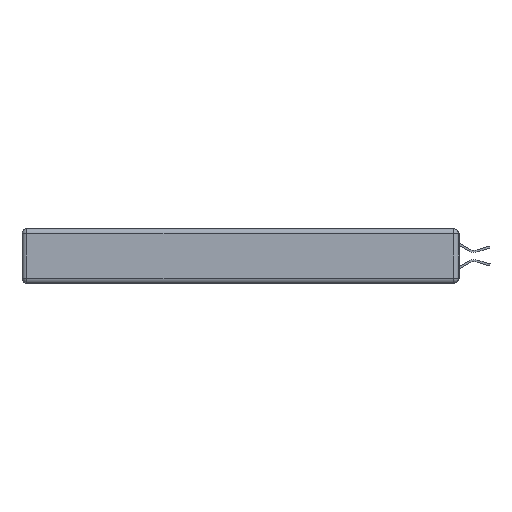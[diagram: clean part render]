
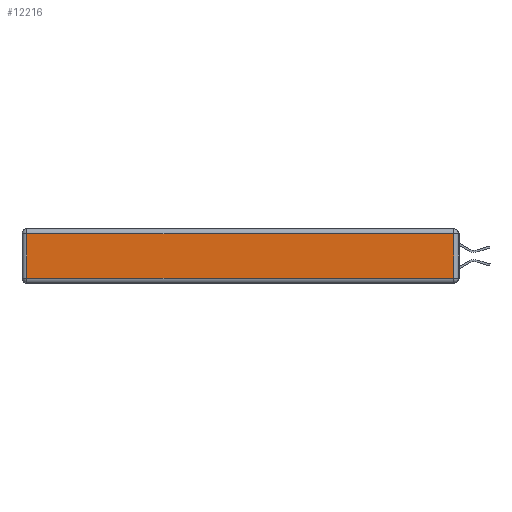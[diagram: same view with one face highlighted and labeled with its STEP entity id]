
A CAD part, left-side view. The second image highlights one B-rep face of the part: STEP entity #12216.
In plain terms, the highlighted planar face has unit normal (-1, 0, 0).
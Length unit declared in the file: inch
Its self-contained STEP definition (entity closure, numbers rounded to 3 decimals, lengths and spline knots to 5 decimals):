
#833 = VERTEX_POINT ( 'NONE', #8917 ) ;
#981 = EDGE_CURVE ( 'NONE', #833, #10644, #5362, .T. ) ;
#1242 = EDGE_CURVE ( 'NONE', #2930, #833, #7885, .T. ) ;
#1251 = CARTESIAN_POINT ( 'NONE',  ( 0., 0., -0.343 ) ) ;
#1290 = DIRECTION ( 'NONE',  ( 0., 1., 0. ) ) ;
#2309 = DIRECTION ( 'NONE',  ( -1., 0., 0. ) ) ;
#2523 = LINE ( 'NONE', #9606, #14091 ) ;
#2930 = VERTEX_POINT ( 'NONE', #4007 ) ;
#4007 = CARTESIAN_POINT ( 'NONE',  ( 0., 0.03, -0.313 ) ) ;
#4127 = CARTESIAN_POINT ( 'NONE',  ( 0., 0.03, -0.343 ) ) ;
#4578 = AXIS2_PLACEMENT_3D ( 'NONE', #1251, #2309, #4764 ) ;
#4607 = PLANE ( 'NONE',  #4578 ) ;
#4764 = DIRECTION ( 'NONE',  ( 0., 0., 1. ) ) ;
#4819 = VERTEX_POINT ( 'NONE', #9860 ) ;
#4936 = FACE_OUTER_BOUND ( 'NONE', #4954, .T. ) ;
#4954 = EDGE_LOOP ( 'NONE', ( #6376, #10042, #5620, #5202 ) ) ;
#5202 = ORIENTED_EDGE ( 'NONE', *, *, #9009, .T. ) ;
#5362 = LINE ( 'NONE', #11624, #5904 ) ;
#5620 = ORIENTED_EDGE ( 'NONE', *, *, #981, .T. ) ;
#5757 = EDGE_CURVE ( 'NONE', #4819, #2930, #2523, .T. ) ;
#5904 = VECTOR ( 'NONE', #1290, 39.37008 ) ;
#6376 = ORIENTED_EDGE ( 'NONE', *, *, #5757, .T. ) ;
#7301 = DIRECTION ( 'NONE',  ( 0., -1., 0. ) ) ;
#7885 = LINE ( 'NONE', #4127, #10228 ) ;
#7890 = CARTESIAN_POINT ( 'NONE',  ( 0., 2.72, -0.343 ) ) ;
#8794 = CARTESIAN_POINT ( 'NONE',  ( 0., 2.72, -0.03 ) ) ;
#8917 = CARTESIAN_POINT ( 'NONE',  ( 0., 0.03, -0.03 ) ) ;
#9009 = EDGE_CURVE ( 'NONE', #10644, #4819, #10794, .T. ) ;
#9606 = CARTESIAN_POINT ( 'NONE',  ( 0., 0., -0.313 ) ) ;
#9860 = CARTESIAN_POINT ( 'NONE',  ( 0., 2.72, -0.313 ) ) ;
#10042 = ORIENTED_EDGE ( 'NONE', *, *, #1242, .T. ) ;
#10228 = VECTOR ( 'NONE', #11352, 39.37008 ) ;
#10644 = VERTEX_POINT ( 'NONE', #8794 ) ;
#10794 = LINE ( 'NONE', #7890, #10963 ) ;
#10963 = VECTOR ( 'NONE', #14627, 39.37008 ) ;
#11352 = DIRECTION ( 'NONE',  ( 0., 0., 1. ) ) ;
#11624 = CARTESIAN_POINT ( 'NONE',  ( 0., 2.75, -0.03 ) ) ;
#12216 = ADVANCED_FACE ( 'NONE', ( #4936 ), #4607, .T. ) ;
#14091 = VECTOR ( 'NONE', #7301, 39.37008 ) ;
#14627 = DIRECTION ( 'NONE',  ( 0., 0., -1. ) ) ;
